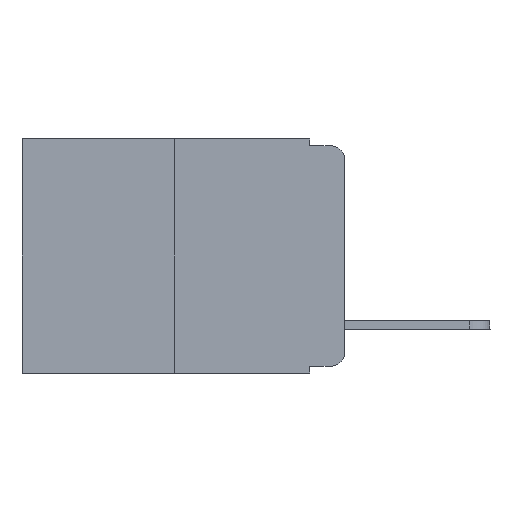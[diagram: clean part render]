
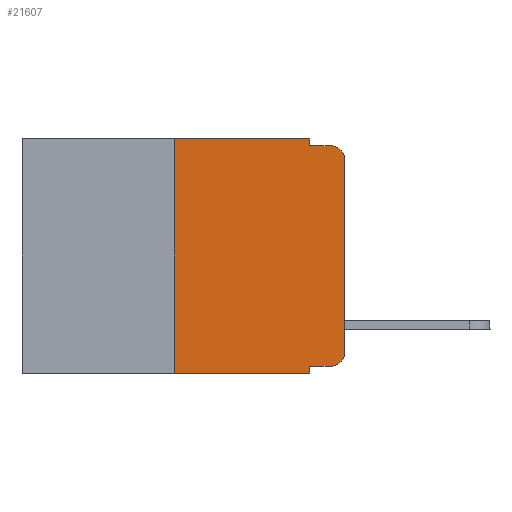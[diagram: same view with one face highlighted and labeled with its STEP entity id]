
A CAD part, left-side view. The second image highlights one B-rep face of the part: STEP entity #21607.
In plain terms, the highlighted planar face has unit normal (-1, 0, 0).
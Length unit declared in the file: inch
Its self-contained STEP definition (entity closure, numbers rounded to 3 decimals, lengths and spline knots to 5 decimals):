
#66 = LINE ( 'NONE', #11824, #2779 ) ;
#192 = DIRECTION ( 'NONE',  ( 0., -1., 0. ) ) ;
#368 = LINE ( 'NONE', #492, #25160 ) ;
#389 = DIRECTION ( 'NONE',  ( 0., 0., -1. ) ) ;
#492 = CARTESIAN_POINT ( 'NONE',  ( 0., 0.051, -0.333 ) ) ;
#683 = LINE ( 'NONE', #20666, #23876 ) ;
#957 = CARTESIAN_POINT ( 'NONE',  ( 0., 0.051, -0.333 ) ) ;
#1272 = ORIENTED_EDGE ( 'NONE', *, *, #7919, .F. ) ;
#2048 = CARTESIAN_POINT ( 'NONE',  ( 0., 0.051, 0. ) ) ;
#2061 = VECTOR ( 'NONE', #23199, 39.37008 ) ;
#2205 = CARTESIAN_POINT ( 'NONE',  ( 0., 0., 0. ) ) ;
#2227 = CIRCLE ( 'NONE', #12244, 0.02 ) ;
#2424 = DIRECTION ( 'NONE',  ( 0., 0., -1. ) ) ;
#2779 = VECTOR ( 'NONE', #9879, 39.37008 ) ;
#2799 = ORIENTED_EDGE ( 'NONE', *, *, #21264, .F. ) ;
#3253 = DIRECTION ( 'NONE',  ( 0., -1., 0. ) ) ;
#3681 = VERTEX_POINT ( 'NONE', #23546 ) ;
#3894 = VERTEX_POINT ( 'NONE', #957 ) ;
#4371 = LINE ( 'NONE', #2048, #22946 ) ;
#4634 = EDGE_CURVE ( 'NONE', #23860, #15291, #22058, .T. ) ;
#5186 = EDGE_CURVE ( 'NONE', #19317, #23860, #22888, .T. ) ;
#5375 = CARTESIAN_POINT ( 'NONE',  ( 0., 0.02, -0.333 ) ) ;
#6501 = DIRECTION ( 'NONE',  ( 0., 0., 1. ) ) ;
#6519 = DIRECTION ( 'NONE',  ( -1., 0., 0. ) ) ;
#6736 = ORIENTED_EDGE ( 'NONE', *, *, #8184, .T. ) ;
#6865 = VERTEX_POINT ( 'NONE', #10296 ) ;
#6956 = CARTESIAN_POINT ( 'NONE',  ( 0., 0., -0.313 ) ) ;
#7155 = LINE ( 'NONE', #9382, #2061 ) ;
#7324 = EDGE_CURVE ( 'NONE', #6865, #18372, #683, .T. ) ;
#7513 = DIRECTION ( 'NONE',  ( 0., 0., -1. ) ) ;
#7919 = EDGE_CURVE ( 'NONE', #3681, #15453, #25171, .T. ) ;
#8184 = EDGE_CURVE ( 'NONE', #3894, #19317, #368, .T. ) ;
#8278 = ORIENTED_EDGE ( 'NONE', *, *, #10256, .T. ) ;
#8655 = ORIENTED_EDGE ( 'NONE', *, *, #20055, .F. ) ;
#8965 = DIRECTION ( 'NONE',  ( 0., 0., -1. ) ) ;
#9328 = CARTESIAN_POINT ( 'NONE',  ( 0., 0.25, -0.343 ) ) ;
#9382 = CARTESIAN_POINT ( 'NONE',  ( 0., 0.051, 0. ) ) ;
#9861 = DIRECTION ( 'NONE',  ( 1., 0., 0. ) ) ;
#9879 = DIRECTION ( 'NONE',  ( 0., -1., 0. ) ) ;
#9990 = VECTOR ( 'NONE', #21649, 39.37008 ) ;
#10256 = EDGE_CURVE ( 'NONE', #24393, #25523, #66, .T. ) ;
#10296 = CARTESIAN_POINT ( 'NONE',  ( 0., 0.25, 0. ) ) ;
#10422 = DIRECTION ( 'NONE',  ( 0., -1., 0. ) ) ;
#10653 = DIRECTION ( 'NONE',  ( -1., 0., 0. ) ) ;
#11202 = ORIENTED_EDGE ( 'NONE', *, *, #5186, .T. ) ;
#11440 = EDGE_CURVE ( 'NONE', #15291, #15453, #2227, .T. ) ;
#11681 = PLANE ( 'NONE',  #14648 ) ;
#11824 = CARTESIAN_POINT ( 'NONE',  ( 0., 0.473, -0.343 ) ) ;
#11876 = CARTESIAN_POINT ( 'NONE',  ( 0., 0.051, -0.343 ) ) ;
#12244 = AXIS2_PLACEMENT_3D ( 'NONE', #20443, #10653, #8965 ) ;
#12439 = ORIENTED_EDGE ( 'NONE', *, *, #7324, .F. ) ;
#12809 = CARTESIAN_POINT ( 'NONE',  ( 0., 0.051, 0. ) ) ;
#13177 = CARTESIAN_POINT ( 'NONE',  ( 0., 0.051, -0.01 ) ) ;
#13681 = CARTESIAN_POINT ( 'NONE',  ( 0., 0.25, 0. ) ) ;
#14038 = EDGE_LOOP ( 'NONE', ( #22687, #20157, #1272, #8655, #12439, #17539, #8278, #2799, #6736, #11202 ) ) ;
#14494 = CARTESIAN_POINT ( 'NONE',  ( 0., 0.02, -0.313 ) ) ;
#14648 = AXIS2_PLACEMENT_3D ( 'NONE', #19638, #9861, #7513 ) ;
#14926 = VECTOR ( 'NONE', #6501, 39.37008 ) ;
#15291 = VERTEX_POINT ( 'NONE', #24616 ) ;
#15453 = VERTEX_POINT ( 'NONE', #17811 ) ;
#17539 = ORIENTED_EDGE ( 'NONE', *, *, #20345, .F. ) ;
#17811 = CARTESIAN_POINT ( 'NONE',  ( 0., 0.02, -0.01 ) ) ;
#18372 = VERTEX_POINT ( 'NONE', #12809 ) ;
#18734 = AXIS2_PLACEMENT_3D ( 'NONE', #14494, #6519, #389 ) ;
#19317 = VERTEX_POINT ( 'NONE', #5375 ) ;
#19344 = VECTOR ( 'NONE', #3253, 39.37008 ) ;
#19638 = CARTESIAN_POINT ( 'NONE',  ( 0., 0.473, 0. ) ) ;
#20055 = EDGE_CURVE ( 'NONE', #18372, #3681, #7155, .T. ) ;
#20071 = LINE ( 'NONE', #13681, #9990 ) ;
#20157 = ORIENTED_EDGE ( 'NONE', *, *, #11440, .T. ) ;
#20345 = EDGE_CURVE ( 'NONE', #24393, #6865, #20071, .T. ) ;
#20443 = CARTESIAN_POINT ( 'NONE',  ( 0., 0.02, -0.03 ) ) ;
#20666 = CARTESIAN_POINT ( 'NONE',  ( 0., 0.473, 0. ) ) ;
#21264 = EDGE_CURVE ( 'NONE', #3894, #25523, #4371, .T. ) ;
#21607 = ADVANCED_FACE ( 'NONE', ( #25502 ), #11681, .F. ) ;
#21649 = DIRECTION ( 'NONE',  ( 0., 0., 1. ) ) ;
#22058 = LINE ( 'NONE', #2205, #14926 ) ;
#22687 = ORIENTED_EDGE ( 'NONE', *, *, #4634, .T. ) ;
#22888 = CIRCLE ( 'NONE', #18734, 0.02 ) ;
#22946 = VECTOR ( 'NONE', #2424, 39.37008 ) ;
#23199 = DIRECTION ( 'NONE',  ( 0., 0., -1. ) ) ;
#23546 = CARTESIAN_POINT ( 'NONE',  ( 0., 0.051, -0.01 ) ) ;
#23860 = VERTEX_POINT ( 'NONE', #6956 ) ;
#23876 = VECTOR ( 'NONE', #192, 39.37008 ) ;
#24393 = VERTEX_POINT ( 'NONE', #9328 ) ;
#24616 = CARTESIAN_POINT ( 'NONE',  ( 0., 0., -0.03 ) ) ;
#25160 = VECTOR ( 'NONE', #10422, 39.37008 ) ;
#25171 = LINE ( 'NONE', #13177, #19344 ) ;
#25502 = FACE_OUTER_BOUND ( 'NONE', #14038, .T. ) ;
#25523 = VERTEX_POINT ( 'NONE', #11876 ) ;
